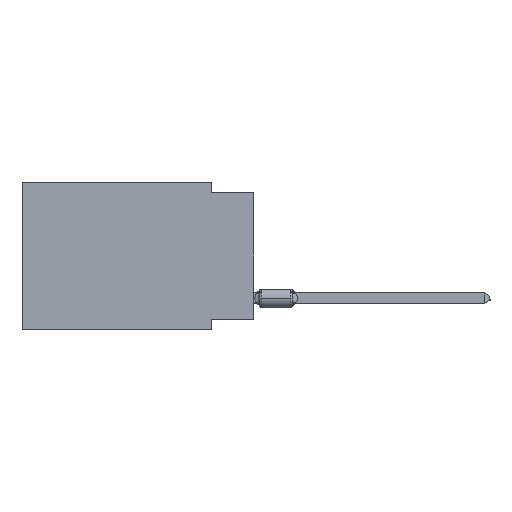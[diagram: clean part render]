
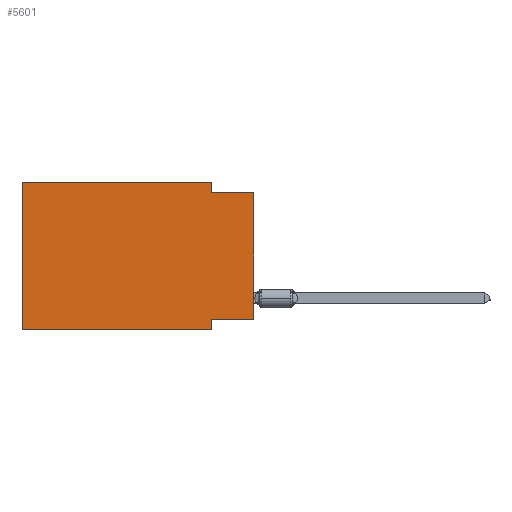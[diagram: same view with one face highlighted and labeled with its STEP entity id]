
A CAD part, left-side view. The second image highlights one B-rep face of the part: STEP entity #5601.
In plain terms, the highlighted planar face has unit normal (-1, 0, 0).
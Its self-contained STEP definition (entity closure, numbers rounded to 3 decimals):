
#300 = LINE ( 'NONE', #16802, #10192 ) ;
#667 = VECTOR ( 'NONE', #20870, 1000. ) ;
#912 = ORIENTED_EDGE ( 'NONE', *, *, #6483, .F. ) ;
#946 = CARTESIAN_POINT ( 'NONE',  ( 0., 2.54, 0. ) ) ;
#1101 = EDGE_CURVE ( 'NONE', #32938, #22506, #5382, .T. ) ;
#1638 = LINE ( 'NONE', #10357, #33187 ) ;
#1885 = CARTESIAN_POINT ( 'NONE',  ( 0., 0., -0.635 ) ) ;
#2159 = CARTESIAN_POINT ( 'NONE',  ( 0., 13.97, -8.89 ) ) ;
#2833 = VECTOR ( 'NONE', #36327, 1000. ) ;
#2885 = DIRECTION ( 'NONE',  ( 0., 1., 0. ) ) ;
#3043 = ORIENTED_EDGE ( 'NONE', *, *, #25544, .F. ) ;
#3645 = LINE ( 'NONE', #31284, #667 ) ;
#3911 = DIRECTION ( 'NONE',  ( 0., 0., -1. ) ) ;
#4219 = CARTESIAN_POINT ( 'NONE',  ( 0., 0., -8.255 ) ) ;
#4435 = PLANE ( 'NONE',  #32557 ) ;
#4714 = CARTESIAN_POINT ( 'NONE',  ( 0., 13.97, 0. ) ) ;
#4778 = DIRECTION ( 'NONE',  ( 0., 0., -1. ) ) ;
#5382 = LINE ( 'NONE', #13543, #2833 ) ;
#5601 = ADVANCED_FACE ( 'NONE', ( #15736 ), #4435, .F. ) ;
#5878 = ORIENTED_EDGE ( 'NONE', *, *, #31491, .T. ) ;
#6483 = EDGE_CURVE ( 'NONE', #32938, #11913, #3645, .T. ) ;
#8295 = ORIENTED_EDGE ( 'NONE', *, *, #30659, .F. ) ;
#8306 = VECTOR ( 'NONE', #3911, 1000. ) ;
#9647 = LINE ( 'NONE', #11857, #8306 ) ;
#10192 = VECTOR ( 'NONE', #2885, 1000. ) ;
#10357 = CARTESIAN_POINT ( 'NONE',  ( 0., 2.54, -8.89 ) ) ;
#10929 = VECTOR ( 'NONE', #20852, 1000. ) ;
#11857 = CARTESIAN_POINT ( 'NONE',  ( 0., 2.54, 0. ) ) ;
#11913 = VERTEX_POINT ( 'NONE', #14582 ) ;
#13285 = EDGE_CURVE ( 'NONE', #26059, #32176, #9647, .T. ) ;
#13543 = CARTESIAN_POINT ( 'NONE',  ( 0., 13.97, -8.89 ) ) ;
#13747 = EDGE_CURVE ( 'NONE', #35280, #22506, #1638, .T. ) ;
#14582 = CARTESIAN_POINT ( 'NONE',  ( 0., 13.97, 0. ) ) ;
#14744 = LINE ( 'NONE', #23627, #10929 ) ;
#15736 = FACE_OUTER_BOUND ( 'NONE', #16723, .T. ) ;
#16723 = EDGE_LOOP ( 'NONE', ( #5878, #3043, #23065, #25497, #912, #28957, #33239, #8295 ) ) ;
#16802 = CARTESIAN_POINT ( 'NONE',  ( 0., 0., -8.255 ) ) ;
#18871 = DIRECTION ( 'NONE',  ( 1., 0., 0. ) ) ;
#20209 = EDGE_CURVE ( 'NONE', #11913, #26059, #30274, .T. ) ;
#20711 = VERTEX_POINT ( 'NONE', #4219 ) ;
#20852 = DIRECTION ( 'NONE',  ( 0., -1., 0. ) ) ;
#20870 = DIRECTION ( 'NONE',  ( 0., 0., 1. ) ) ;
#22506 = VERTEX_POINT ( 'NONE', #31634 ) ;
#23065 = ORIENTED_EDGE ( 'NONE', *, *, #13285, .F. ) ;
#23627 = CARTESIAN_POINT ( 'NONE',  ( 0., 0., -0.635 ) ) ;
#24640 = CARTESIAN_POINT ( 'NONE',  ( 0., 13.97, 0. ) ) ;
#25024 = CARTESIAN_POINT ( 'NONE',  ( 0., 2.54, -0.635 ) ) ;
#25497 = ORIENTED_EDGE ( 'NONE', *, *, #20209, .F. ) ;
#25544 = EDGE_CURVE ( 'NONE', #32176, #29791, #14744, .T. ) ;
#25886 = CARTESIAN_POINT ( 'NONE',  ( 0., 0., 0. ) ) ;
#26059 = VERTEX_POINT ( 'NONE', #946 ) ;
#28957 = ORIENTED_EDGE ( 'NONE', *, *, #1101, .T. ) ;
#29791 = VERTEX_POINT ( 'NONE', #1885 ) ;
#30168 = DIRECTION ( 'NONE',  ( 0., 0., -1. ) ) ;
#30274 = LINE ( 'NONE', #4714, #36385 ) ;
#30659 = EDGE_CURVE ( 'NONE', #20711, #35280, #300, .T. ) ;
#30941 = VECTOR ( 'NONE', #34213, 1000. ) ;
#31284 = CARTESIAN_POINT ( 'NONE',  ( 0., 13.97, 0. ) ) ;
#31491 = EDGE_CURVE ( 'NONE', #20711, #29791, #31615, .T. ) ;
#31615 = LINE ( 'NONE', #25886, #30941 ) ;
#31634 = CARTESIAN_POINT ( 'NONE',  ( 0., 2.54, -8.89 ) ) ;
#32040 = CARTESIAN_POINT ( 'NONE',  ( 0., 2.54, -8.255 ) ) ;
#32176 = VERTEX_POINT ( 'NONE', #25024 ) ;
#32557 = AXIS2_PLACEMENT_3D ( 'NONE', #24640, #18871, #30168 ) ;
#32938 = VERTEX_POINT ( 'NONE', #2159 ) ;
#33187 = VECTOR ( 'NONE', #4778, 1000. ) ;
#33239 = ORIENTED_EDGE ( 'NONE', *, *, #13747, .F. ) ;
#34213 = DIRECTION ( 'NONE',  ( 0., 0., 1. ) ) ;
#35280 = VERTEX_POINT ( 'NONE', #32040 ) ;
#35855 = DIRECTION ( 'NONE',  ( 0., -1., 0. ) ) ;
#36327 = DIRECTION ( 'NONE',  ( 0., -1., 0. ) ) ;
#36385 = VECTOR ( 'NONE', #35855, 1000. ) ;
